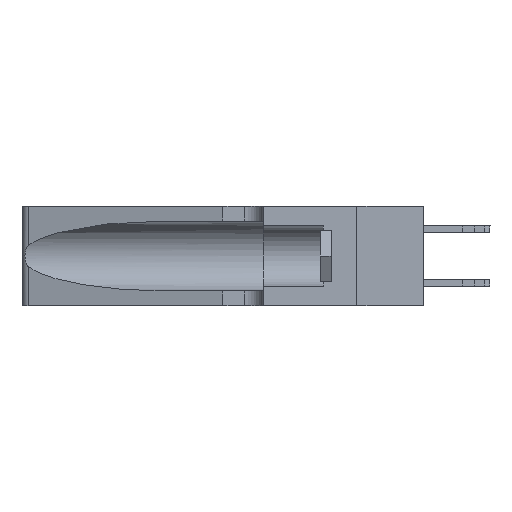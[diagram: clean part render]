
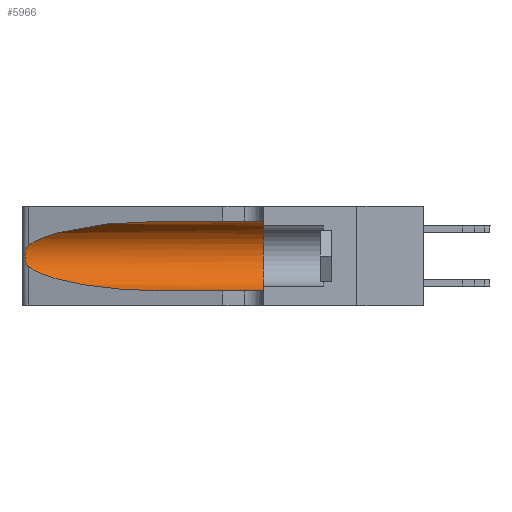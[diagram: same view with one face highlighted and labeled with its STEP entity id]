
A CAD part, left-side view. The second image highlights one B-rep face of the part: STEP entity #5966.
In plain terms, the highlighted cylindrical face has radius 3.308 mm (diameter 6.617 mm), a partial arc.
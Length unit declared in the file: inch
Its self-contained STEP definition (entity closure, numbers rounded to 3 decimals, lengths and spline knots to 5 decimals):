
#281 = CARTESIAN_POINT ( 'NONE',  ( 0.1305, 0.35, 0.31525 ) ) ;
#562 = CARTESIAN_POINT ( 'NONE',  ( 0.26018, 1.23835, 0.19895 ) ) ;
#637 = CARTESIAN_POINT ( 'NONE',  ( 0.26075, 1.23896, 0.178 ) ) ;
#737 = CARTESIAN_POINT ( 'NONE',  ( 0.2373, 1.15595, 0.28018 ) ) ;
#771 = CARTESIAN_POINT ( 'NONE',  ( 0.1305, 1.61858, 0.31525 ) ) ;
#805 = CARTESIAN_POINT ( 'NONE',  ( 0.25555, 1.22994, 0.2215 ) ) ;
#1301 = EDGE_CURVE ( 'NONE', #3985, #18547, #15995, .T. ) ;
#1655 = FACE_OUTER_BOUND ( 'NONE', #14680, .T. ) ;
#1740 = CARTESIAN_POINT ( 'NONE',  ( 0.25487, 1.22718, 0.14631 ) ) ;
#1887 = CARTESIAN_POINT ( 'NONE',  ( 0.1305, 0.72297, 0.05475 ) ) ;
#1957 = VECTOR ( 'NONE', #5014, 39.37008 ) ;
#2384 = CARTESIAN_POINT ( 'NONE',  ( 0.25555, 1.22993, 0.14849 ) ) ;
#2994 = VERTEX_POINT ( 'NONE', #18199 ) ;
#3162 = ORIENTED_EDGE ( 'NONE', *, *, #1301, .T. ) ;
#3278 = VERTEX_POINT ( 'NONE', #281 ) ;
#3546 = CARTESIAN_POINT ( 'NONE',  ( 0.25487, 1.22718, 0.22369 ) ) ;
#3637 = LINE ( 'NONE', #15502, #1957 ) ;
#3985 = VERTEX_POINT ( 'NONE', #1740 ) ;
#4137 = DIRECTION ( 'NONE',  ( 0., 0., 1. ) ) ;
#4274 = CARTESIAN_POINT ( 'NONE',  ( 0.1305, 0.72297, 0.31525 ) ) ;
#4418 = CARTESIAN_POINT ( 'NONE',  ( 0.25487, 1.22718, 0.14631 ) ) ;
#4513 = B_SPLINE_CURVE_WITH_KNOTS ( 'NONE', 3,
 ( #14822, #805, #7491, #7568, #19865, #562, #11075, #637, #19951, #18164, #5931, #19798, #2384, #16427 ),
 .UNSPECIFIED., .F., .F.,
 ( 4, 2, 2, 2, 2, 2, 4 ),
 ( 0., 0.00027, 0.00053, 0.00107, 0.0016, 0.00187, 0.00214 ),
 .UNSPECIFIED. ) ;
#5014 = DIRECTION ( 'NONE',  ( 0., -1., 0. ) ) ;
#5639 = ORIENTED_EDGE ( 'NONE', *, *, #7129, .F. ) ;
#5711 = ORIENTED_EDGE ( 'NONE', *, *, #10344, .F. ) ;
#5931 = CARTESIAN_POINT ( 'NONE',  ( 0.25789, 1.23486, 0.15765 ) ) ;
#5966 = ADVANCED_FACE ( 'NONE', ( #1655 ), #6028, .F. ) ;
#6028 = CYLINDRICAL_SURFACE ( 'NONE', #18437, 0.13025 ) ;
#6265 = EDGE_CURVE ( 'NONE', #21596, #3985, #4513, .T. ) ;
#6810 = CIRCLE ( 'NONE', #21046, 0.13025 ) ;
#7129 = EDGE_CURVE ( 'NONE', #21671, #3278, #10490, .T. ) ;
#7491 = CARTESIAN_POINT ( 'NONE',  ( 0.25639, 1.23184, 0.21858 ) ) ;
#7568 = CARTESIAN_POINT ( 'NONE',  ( 0.25787, 1.23484, 0.2124 ) ) ;
#8253 =( BOUNDED_CURVE ( )  B_SPLINE_CURVE ( 3, ( #4274, #21818, #737, #16360 ),
 .UNSPECIFIED., .F., .T. ) 
 B_SPLINE_CURVE_WITH_KNOTS ( ( 4, 4 ),
 ( 1.5708, 2.84003 ),
 .UNSPECIFIED. ) 
 CURVE ( )  GEOMETRIC_REPRESENTATION_ITEM ( )  RATIONAL_B_SPLINE_CURVE ( ( 1., 0.87, 0.87, 1. ) ) 
 REPRESENTATION_ITEM ( '' )  );
#8315 = ORIENTED_EDGE ( 'NONE', *, *, #6265, .T. ) ;
#8925 = CARTESIAN_POINT ( 'NONE',  ( 0.1305, 0.72297, 0.31525 ) ) ;
#9135 = ORIENTED_EDGE ( 'NONE', *, *, #16042, .T. ) ;
#10344 = EDGE_CURVE ( 'NONE', #3278, #2994, #6810, .T. ) ;
#10490 = LINE ( 'NONE', #771, #18466 ) ;
#11075 = CARTESIAN_POINT ( 'NONE',  ( 0.26075, 1.23896, 0.19203 ) ) ;
#11785 = CARTESIAN_POINT ( 'NONE',  ( 0.1305, 0.72297, 0.05475 ) ) ;
#12302 = DIRECTION ( 'NONE',  ( 0., 1., 0. ) ) ;
#13547 = CARTESIAN_POINT ( 'NONE',  ( 0.1305, 1.61858, 0.185 ) ) ;
#13942 = DIRECTION ( 'NONE',  ( 0., 0., -1. ) ) ;
#14680 = EDGE_LOOP ( 'NONE', ( #16150, #8315, #3162, #9135, #5711, #5639 ) ) ;
#14822 = CARTESIAN_POINT ( 'NONE',  ( 0.25487, 1.22718, 0.22369 ) ) ;
#15502 = CARTESIAN_POINT ( 'NONE',  ( 0.1305, 1.61858, 0.05475 ) ) ;
#15995 =( BOUNDED_CURVE ( )  B_SPLINE_CURVE ( 3, ( #4418, #16655, #20184, #11785 ),
 .UNSPECIFIED., .F., .T. ) 
 B_SPLINE_CURVE_WITH_KNOTS ( ( 4, 4 ),
 ( 3.44316, 4.71239 ),
 .UNSPECIFIED. ) 
 CURVE ( )  GEOMETRIC_REPRESENTATION_ITEM ( )  RATIONAL_B_SPLINE_CURVE ( ( 1., 0.87, 0.87, 1. ) ) 
 REPRESENTATION_ITEM ( '' )  );
#16042 = EDGE_CURVE ( 'NONE', #18547, #2994, #3637, .T. ) ;
#16150 = ORIENTED_EDGE ( 'NONE', *, *, #18686, .T. ) ;
#16360 = CARTESIAN_POINT ( 'NONE',  ( 0.25487, 1.22718, 0.22369 ) ) ;
#16427 = CARTESIAN_POINT ( 'NONE',  ( 0.25487, 1.22718, 0.14631 ) ) ;
#16543 = DIRECTION ( 'NONE',  ( 0., -1., 0. ) ) ;
#16655 = CARTESIAN_POINT ( 'NONE',  ( 0.2373, 1.15595, 0.08982 ) ) ;
#18164 = CARTESIAN_POINT ( 'NONE',  ( 0.25856, 1.23593, 0.16098 ) ) ;
#18199 = CARTESIAN_POINT ( 'NONE',  ( 0.1305, 0.35, 0.05475 ) ) ;
#18437 = AXIS2_PLACEMENT_3D ( 'NONE', #13547, #21156, #13942 ) ;
#18466 = VECTOR ( 'NONE', #16543, 39.37008 ) ;
#18547 = VERTEX_POINT ( 'NONE', #1887 ) ;
#18686 = EDGE_CURVE ( 'NONE', #21671, #21596, #8253, .T. ) ;
#19632 = CARTESIAN_POINT ( 'NONE',  ( 0.1305, 0.35, 0.185 ) ) ;
#19798 = CARTESIAN_POINT ( 'NONE',  ( 0.25639, 1.23186, 0.15144 ) ) ;
#19865 = CARTESIAN_POINT ( 'NONE',  ( 0.25854, 1.2359, 0.20912 ) ) ;
#19951 = CARTESIAN_POINT ( 'NONE',  ( 0.26017, 1.23833, 0.17102 ) ) ;
#20184 = CARTESIAN_POINT ( 'NONE',  ( 0.18966, 0.96281, 0.05475 ) ) ;
#21046 = AXIS2_PLACEMENT_3D ( 'NONE', #19632, #12302, #4137 ) ;
#21156 = DIRECTION ( 'NONE',  ( 0., -1., 0. ) ) ;
#21596 = VERTEX_POINT ( 'NONE', #3546 ) ;
#21671 = VERTEX_POINT ( 'NONE', #8925 ) ;
#21818 = CARTESIAN_POINT ( 'NONE',  ( 0.18966, 0.96281, 0.31525 ) ) ;
